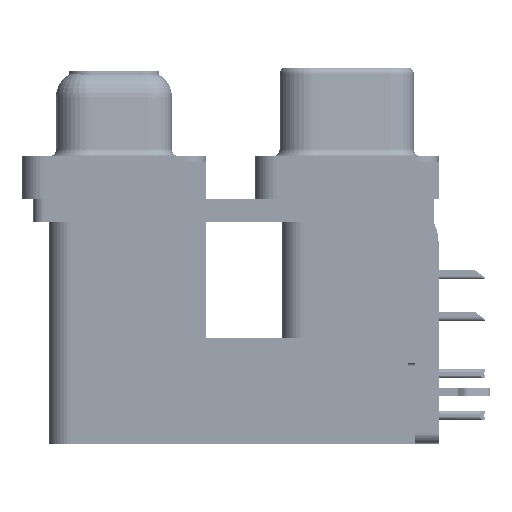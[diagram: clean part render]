
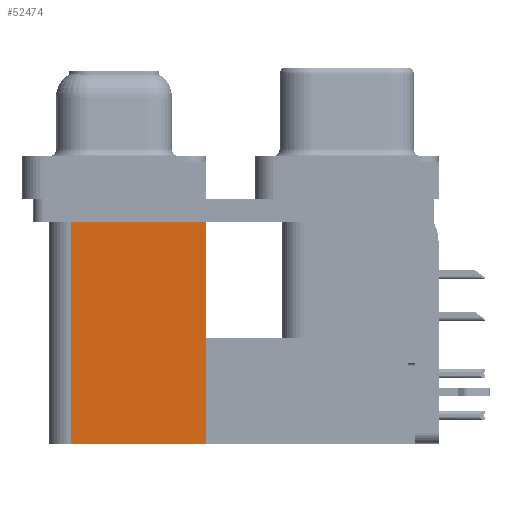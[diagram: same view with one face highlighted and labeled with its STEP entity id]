
A CAD part, left-side view. The second image highlights one B-rep face of the part: STEP entity #52474.
In plain terms, the highlighted planar face has unit normal (-1, 0, 0).
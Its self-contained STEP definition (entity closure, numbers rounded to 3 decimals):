
#2059 = VERTEX_POINT ( 'NONE', #58837 ) ;
#3249 = ORIENTED_EDGE ( 'NONE', *, *, #38079, .F. ) ;
#8654 = CARTESIAN_POINT ( 'NONE',  ( 3.79, 9.6, -2.5 ) ) ;
#8764 = ORIENTED_EDGE ( 'NONE', *, *, #66719, .T. ) ;
#9760 = LINE ( 'NONE', #31204, #36795 ) ;
#10092 = DIRECTION ( 'NONE',  ( 0., 1., 0. ) ) ;
#10532 = PLANE ( 'NONE',  #33356 ) ;
#11081 = CARTESIAN_POINT ( 'NONE',  ( 3.79, 9.6, -19.2 ) ) ;
#11492 = VECTOR ( 'NONE', #20074, 1000. ) ;
#12026 = ORIENTED_EDGE ( 'NONE', *, *, #19480, .F. ) ;
#14785 = DIRECTION ( 'NONE',  ( 0., 1., 0. ) ) ;
#19480 = EDGE_CURVE ( 'NONE', #22239, #2059, #35543, .T. ) ;
#20074 = DIRECTION ( 'NONE',  ( 0., 1., 0. ) ) ;
#21298 = LINE ( 'NONE', #11081, #25669 ) ;
#22239 = VERTEX_POINT ( 'NONE', #54001 ) ;
#24971 = DIRECTION ( 'NONE',  ( 0., 0., 1. ) ) ;
#25402 = ORIENTED_EDGE ( 'NONE', *, *, #29189, .T. ) ;
#25669 = VECTOR ( 'NONE', #58618, 1000. ) ;
#29189 = EDGE_CURVE ( 'NONE', #49369, #2059, #56715, .T. ) ;
#31204 = CARTESIAN_POINT ( 'NONE',  ( 3.79, 9.6, -19.2 ) ) ;
#33356 = AXIS2_PLACEMENT_3D ( 'NONE', #36924, #46836, #14785 ) ;
#35543 = LINE ( 'NONE', #57041, #50924 ) ;
#36795 = VECTOR ( 'NONE', #10092, 1000. ) ;
#36924 = CARTESIAN_POINT ( 'NONE',  ( 3.79, 9.6, -19.2 ) ) ;
#38079 = EDGE_CURVE ( 'NONE', #68234, #22239, #9760, .T. ) ;
#41186 = FACE_OUTER_BOUND ( 'NONE', #69238, .T. ) ;
#46836 = DIRECTION ( 'NONE',  ( 1., 0., 0. ) ) ;
#49369 = VERTEX_POINT ( 'NONE', #8654 ) ;
#50718 = CARTESIAN_POINT ( 'NONE',  ( 3.79, 9.6, -2.5 ) ) ;
#50846 = CARTESIAN_POINT ( 'NONE',  ( 3.79, 9.6, -19.2 ) ) ;
#50924 = VECTOR ( 'NONE', #24971, 1000. ) ;
#52474 = ADVANCED_FACE ( 'NONE', ( #41186 ), #10532, .F. ) ;
#54001 = CARTESIAN_POINT ( 'NONE',  ( 3.79, 18.8, -19.2 ) ) ;
#56715 = LINE ( 'NONE', #50718, #11492 ) ;
#57041 = CARTESIAN_POINT ( 'NONE',  ( 3.79, 18.8, -19.2 ) ) ;
#58618 = DIRECTION ( 'NONE',  ( 0., 0., 1. ) ) ;
#58837 = CARTESIAN_POINT ( 'NONE',  ( 3.79, 18.8, -2.5 ) ) ;
#66719 = EDGE_CURVE ( 'NONE', #68234, #49369, #21298, .T. ) ;
#68234 = VERTEX_POINT ( 'NONE', #50846 ) ;
#69238 = EDGE_LOOP ( 'NONE', ( #25402, #12026, #3249, #8764 ) ) ;
